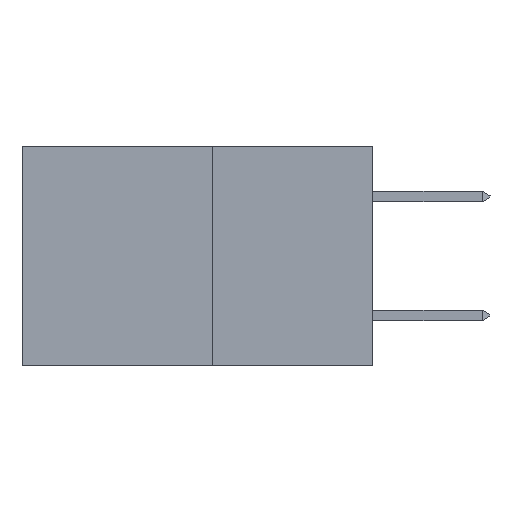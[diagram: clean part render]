
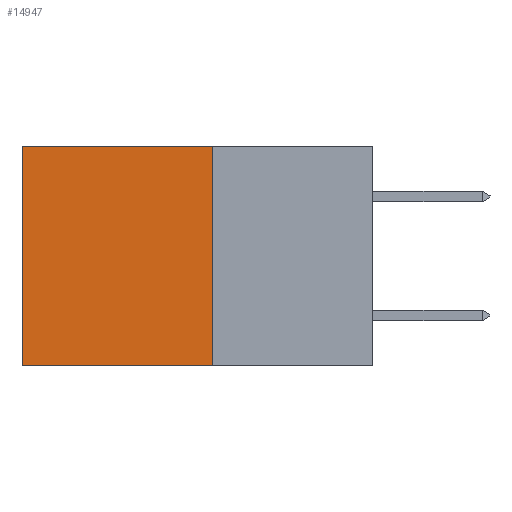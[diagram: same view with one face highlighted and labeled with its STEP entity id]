
A CAD part, left-side view. The second image highlights one B-rep face of the part: STEP entity #14947.
In plain terms, the highlighted planar face has unit normal (-1, 0, 0).
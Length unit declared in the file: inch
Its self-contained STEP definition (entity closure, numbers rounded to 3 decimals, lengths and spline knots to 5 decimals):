
#225 = CARTESIAN_POINT ( 'NONE',  ( 0.277, 0.59, 0. ) ) ;
#315 = LINE ( 'NONE', #6194, #8116 ) ;
#490 = EDGE_CURVE ( 'NONE', #1608, #11492, #20759, .T. ) ;
#895 = VERTEX_POINT ( 'NONE', #225 ) ;
#1608 = VERTEX_POINT ( 'NONE', #11156 ) ;
#3368 = ORIENTED_EDGE ( 'NONE', *, *, #8351, .F. ) ;
#3832 = EDGE_CURVE ( 'NONE', #895, #18044, #315, .T. ) ;
#4717 = ORIENTED_EDGE ( 'NONE', *, *, #490, .F. ) ;
#6093 = PLANE ( 'NONE',  #20747 ) ;
#6138 = DIRECTION ( 'NONE',  ( 0., 0., -1. ) ) ;
#6194 = CARTESIAN_POINT ( 'NONE',  ( 0.277, 0.59, -0.37 ) ) ;
#6353 = VECTOR ( 'NONE', #15124, 39.37008 ) ;
#6363 = FACE_OUTER_BOUND ( 'NONE', #10227, .T. ) ;
#7798 = VECTOR ( 'NONE', #9329, 39.37008 ) ;
#8116 = VECTOR ( 'NONE', #6138, 39.37008 ) ;
#8170 = VECTOR ( 'NONE', #10661, 39.37008 ) ;
#8335 = LINE ( 'NONE', #20073, #7798 ) ;
#8351 = EDGE_CURVE ( 'NONE', #11492, #18044, #8335, .T. ) ;
#9329 = DIRECTION ( 'NONE',  ( 0., 1., 0. ) ) ;
#10227 = EDGE_LOOP ( 'NONE', ( #12070, #3368, #4717, #16138 ) ) ;
#10661 = DIRECTION ( 'NONE',  ( 0., 0., -1. ) ) ;
#11156 = CARTESIAN_POINT ( 'NONE',  ( 0.277, 0.27, 0. ) ) ;
#11351 = CARTESIAN_POINT ( 'NONE',  ( 0.277, 0.59, -0.37 ) ) ;
#11492 = VERTEX_POINT ( 'NONE', #15757 ) ;
#12070 = ORIENTED_EDGE ( 'NONE', *, *, #3832, .T. ) ;
#12585 = EDGE_CURVE ( 'NONE', #1608, #895, #19065, .T. ) ;
#13854 = CARTESIAN_POINT ( 'NONE',  ( 0.277, 0.27, -0.37 ) ) ;
#14947 = ADVANCED_FACE ( 'NONE', ( #6363 ), #6093, .F. ) ;
#15124 = DIRECTION ( 'NONE',  ( 0., 1., 0. ) ) ;
#15757 = CARTESIAN_POINT ( 'NONE',  ( 0.277, 0.27, -0.37 ) ) ;
#16138 = ORIENTED_EDGE ( 'NONE', *, *, #12585, .T. ) ;
#16587 = DIRECTION ( 'NONE',  ( 0., 0., -1. ) ) ;
#16664 = DIRECTION ( 'NONE',  ( 1., 0., 0. ) ) ;
#18044 = VERTEX_POINT ( 'NONE', #11351 ) ;
#18801 = CARTESIAN_POINT ( 'NONE',  ( 0.277, 0.27, 0. ) ) ;
#19065 = LINE ( 'NONE', #18801, #6353 ) ;
#19686 = CARTESIAN_POINT ( 'NONE',  ( 0.277, 0.27, -0.37 ) ) ;
#20073 = CARTESIAN_POINT ( 'NONE',  ( 0.277, 0.27, -0.37 ) ) ;
#20747 = AXIS2_PLACEMENT_3D ( 'NONE', #13854, #16664, #16587 ) ;
#20759 = LINE ( 'NONE', #19686, #8170 ) ;
